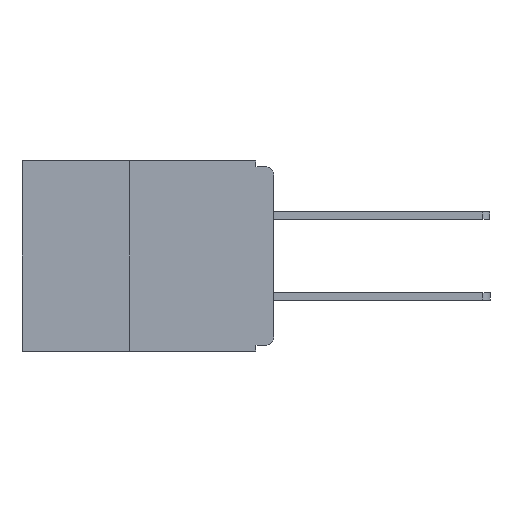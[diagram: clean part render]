
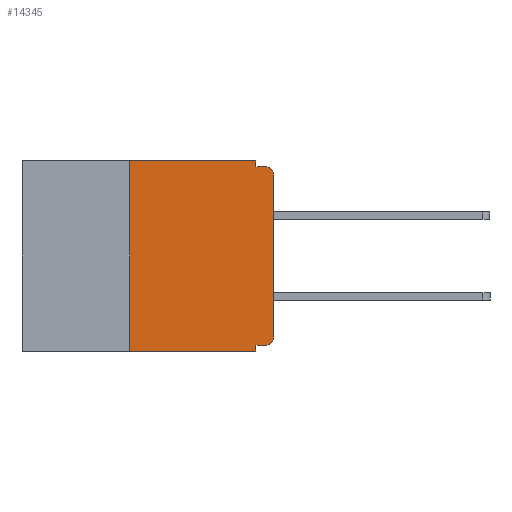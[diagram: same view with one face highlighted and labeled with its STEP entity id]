
A CAD part, left-side view. The second image highlights one B-rep face of the part: STEP entity #14345.
In plain terms, the highlighted planar face has unit normal (-1, 0, 0).
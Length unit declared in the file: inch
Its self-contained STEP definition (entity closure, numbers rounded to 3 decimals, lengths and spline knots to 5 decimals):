
#110 = VERTEX_POINT ( 'NONE', #2596 ) ;
#357 = CARTESIAN_POINT ( 'NONE',  ( 0., 0.031, -0.32 ) ) ;
#1123 = LINE ( 'NONE', #13495, #12738 ) ;
#1372 = EDGE_CURVE ( 'NONE', #12284, #9759, #7779, .T. ) ;
#1534 = VERTEX_POINT ( 'NONE', #10324 ) ;
#1691 = LINE ( 'NONE', #9526, #14015 ) ;
#2208 = VERTEX_POINT ( 'NONE', #9957 ) ;
#2374 = ORIENTED_EDGE ( 'NONE', *, *, #11386, .F. ) ;
#2406 = EDGE_CURVE ( 'NONE', #1534, #2795, #15249, .T. ) ;
#2559 = ORIENTED_EDGE ( 'NONE', *, *, #10045, .T. ) ;
#2596 = CARTESIAN_POINT ( 'NONE',  ( 0., 0.25, -0.33 ) ) ;
#2763 = ORIENTED_EDGE ( 'NONE', *, *, #12473, .F. ) ;
#2795 = VERTEX_POINT ( 'NONE', #11808 ) ;
#2861 = LINE ( 'NONE', #5824, #11651 ) ;
#2922 = CARTESIAN_POINT ( 'NONE',  ( 0., 0.437, -0.33 ) ) ;
#3028 = PLANE ( 'NONE',  #5871 ) ;
#3101 = VERTEX_POINT ( 'NONE', #357 ) ;
#3205 = CARTESIAN_POINT ( 'NONE',  ( 0., 0.437, 0. ) ) ;
#3211 = LINE ( 'NONE', #3205, #15046 ) ;
#3259 = DIRECTION ( 'NONE',  ( 0., -1., 0. ) ) ;
#3734 = DIRECTION ( 'NONE',  ( 0., 0., -1. ) ) ;
#3832 = EDGE_CURVE ( 'NONE', #9759, #2208, #1691, .T. ) ;
#4004 = DIRECTION ( 'NONE',  ( 0., 0., 1. ) ) ;
#4267 = DIRECTION ( 'NONE',  ( 0., 0., -1. ) ) ;
#4486 = ORIENTED_EDGE ( 'NONE', *, *, #12827, .F. ) ;
#4606 = VECTOR ( 'NONE', #6999, 39.37008 ) ;
#4652 = EDGE_CURVE ( 'NONE', #12497, #12284, #3211, .T. ) ;
#5198 = DIRECTION ( 'NONE',  ( 0., 0., 1. ) ) ;
#5824 = CARTESIAN_POINT ( 'NONE',  ( 0., 0., -0.32 ) ) ;
#5871 = AXIS2_PLACEMENT_3D ( 'NONE', #7815, #11406, #4267 ) ;
#5961 = LINE ( 'NONE', #6402, #8779 ) ;
#5968 = ORIENTED_EDGE ( 'NONE', *, *, #2406, .T. ) ;
#6160 = ORIENTED_EDGE ( 'NONE', *, *, #7237, .T. ) ;
#6402 = CARTESIAN_POINT ( 'NONE',  ( 0., 0., 0. ) ) ;
#6683 = CARTESIAN_POINT ( 'NONE',  ( 0., 0.031, 0. ) ) ;
#6901 = CARTESIAN_POINT ( 'NONE',  ( 0., 0.015, -0.025 ) ) ;
#6999 = DIRECTION ( 'NONE',  ( 0., 0., -1. ) ) ;
#7016 = VERTEX_POINT ( 'NONE', #13896 ) ;
#7053 = DIRECTION ( 'NONE',  ( 0., 1., 0. ) ) ;
#7237 = EDGE_CURVE ( 'NONE', #7016, #2208, #7669, .T. ) ;
#7669 = CIRCLE ( 'NONE', #10931, 0.015 ) ;
#7779 = LINE ( 'NONE', #14553, #4606 ) ;
#7815 = CARTESIAN_POINT ( 'NONE',  ( 0., 0.437, 0. ) ) ;
#7975 = LINE ( 'NONE', #10894, #14233 ) ;
#8010 = CARTESIAN_POINT ( 'NONE',  ( 0., 0.031, -0.33 ) ) ;
#8114 = DIRECTION ( 'NONE',  ( 0., 0., -1. ) ) ;
#8779 = VECTOR ( 'NONE', #5198, 39.37008 ) ;
#8991 = FACE_OUTER_BOUND ( 'NONE', #13587, .T. ) ;
#9033 = VERTEX_POINT ( 'NONE', #8010 ) ;
#9496 = DIRECTION ( 'NONE',  ( 0., -1., 0. ) ) ;
#9526 = CARTESIAN_POINT ( 'NONE',  ( 0., 0., -0.01 ) ) ;
#9741 = LINE ( 'NONE', #2922, #13244 ) ;
#9759 = VERTEX_POINT ( 'NONE', #12963 ) ;
#9957 = CARTESIAN_POINT ( 'NONE',  ( 0., 0.015, -0.01 ) ) ;
#10045 = EDGE_CURVE ( 'NONE', #2795, #7016, #5961, .T. ) ;
#10092 = ORIENTED_EDGE ( 'NONE', *, *, #3832, .F. ) ;
#10324 = CARTESIAN_POINT ( 'NONE',  ( 0., 0.015, -0.32 ) ) ;
#10467 = ORIENTED_EDGE ( 'NONE', *, *, #4652, .F. ) ;
#10659 = CARTESIAN_POINT ( 'NONE',  ( 0., 0.25, 0. ) ) ;
#10687 = AXIS2_PLACEMENT_3D ( 'NONE', #15110, #14973, #14718 ) ;
#10894 = CARTESIAN_POINT ( 'NONE',  ( 0., 0.031, -0.33 ) ) ;
#10931 = AXIS2_PLACEMENT_3D ( 'NONE', #6901, #15109, #8114 ) ;
#11299 = DIRECTION ( 'NONE',  ( 0., -1., 0. ) ) ;
#11386 = EDGE_CURVE ( 'NONE', #3101, #9033, #7975, .T. ) ;
#11406 = DIRECTION ( 'NONE',  ( 1., 0., 0. ) ) ;
#11651 = VECTOR ( 'NONE', #7053, 39.37008 ) ;
#11808 = CARTESIAN_POINT ( 'NONE',  ( 0., 0., -0.305 ) ) ;
#12284 = VERTEX_POINT ( 'NONE', #6683 ) ;
#12473 = EDGE_CURVE ( 'NONE', #1534, #3101, #2861, .T. ) ;
#12497 = VERTEX_POINT ( 'NONE', #10659 ) ;
#12738 = VECTOR ( 'NONE', #4004, 39.37008 ) ;
#12827 = EDGE_CURVE ( 'NONE', #110, #12497, #1123, .T. ) ;
#12963 = CARTESIAN_POINT ( 'NONE',  ( 0., 0.031, -0.01 ) ) ;
#13220 = ORIENTED_EDGE ( 'NONE', *, *, #1372, .F. ) ;
#13244 = VECTOR ( 'NONE', #11299, 39.37008 ) ;
#13495 = CARTESIAN_POINT ( 'NONE',  ( 0., 0.25, -0.33 ) ) ;
#13587 = EDGE_LOOP ( 'NONE', ( #2559, #6160, #10092, #13220, #10467, #4486, #14632, #2374, #2763, #5968 ) ) ;
#13896 = CARTESIAN_POINT ( 'NONE',  ( 0., 0., -0.025 ) ) ;
#14015 = VECTOR ( 'NONE', #9496, 39.37008 ) ;
#14233 = VECTOR ( 'NONE', #3734, 39.37008 ) ;
#14280 = EDGE_CURVE ( 'NONE', #110, #9033, #9741, .T. ) ;
#14345 = ADVANCED_FACE ( 'NONE', ( #8991 ), #3028, .F. ) ;
#14553 = CARTESIAN_POINT ( 'NONE',  ( 0., 0.031, 0. ) ) ;
#14632 = ORIENTED_EDGE ( 'NONE', *, *, #14280, .T. ) ;
#14718 = DIRECTION ( 'NONE',  ( 0., 0., -1. ) ) ;
#14973 = DIRECTION ( 'NONE',  ( -1., 0., 0. ) ) ;
#15046 = VECTOR ( 'NONE', #3259, 39.37008 ) ;
#15109 = DIRECTION ( 'NONE',  ( -1., 0., 0. ) ) ;
#15110 = CARTESIAN_POINT ( 'NONE',  ( 0., 0.015, -0.305 ) ) ;
#15249 = CIRCLE ( 'NONE', #10687, 0.015 ) ;
